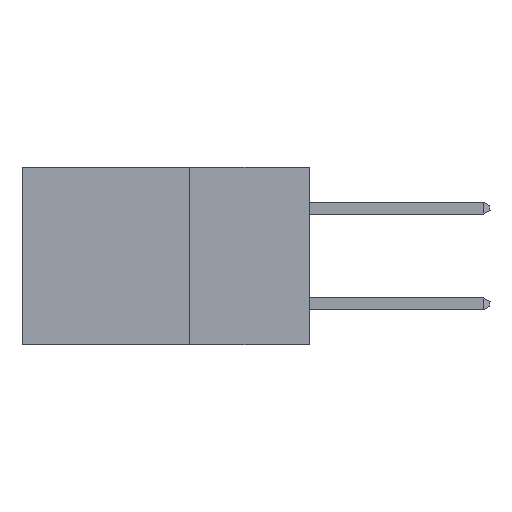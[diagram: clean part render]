
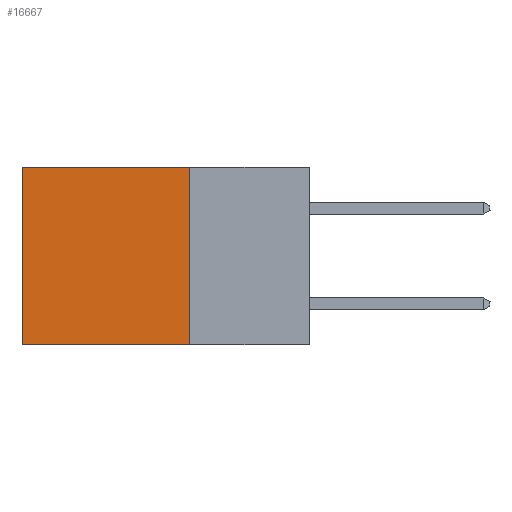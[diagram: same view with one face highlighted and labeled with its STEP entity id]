
A CAD part, left-side view. The second image highlights one B-rep face of the part: STEP entity #16667.
In plain terms, the highlighted planar face has unit normal (-1, 0, 0).
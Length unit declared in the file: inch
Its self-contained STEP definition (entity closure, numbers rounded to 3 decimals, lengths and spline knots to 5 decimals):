
#1924 = DIRECTION ( 'NONE',  ( 0., 0., -1. ) ) ;
#2074 = CARTESIAN_POINT ( 'NONE',  ( 0.2875, 0.25, 0. ) ) ;
#3397 = VECTOR ( 'NONE', #35316, 39.37008 ) ;
#5446 = EDGE_CURVE ( 'NONE', #33733, #5784, #24903, .T. ) ;
#5784 = VERTEX_POINT ( 'NONE', #41349 ) ;
#9668 = DIRECTION ( 'NONE',  ( 1., 0., 0. ) ) ;
#10175 = VECTOR ( 'NONE', #28553, 39.37008 ) ;
#13163 = VECTOR ( 'NONE', #1924, 39.37008 ) ;
#13695 = DIRECTION ( 'NONE',  ( 0., 0., -1. ) ) ;
#14239 = EDGE_CURVE ( 'NONE', #25589, #33733, #38226, .T. ) ;
#14342 = LINE ( 'NONE', #14588, #3397 ) ;
#14551 = CARTESIAN_POINT ( 'NONE',  ( 0.2875, 0.25, -0.37 ) ) ;
#14588 = CARTESIAN_POINT ( 'NONE',  ( 0.2875, 0.25, 0. ) ) ;
#16606 = VERTEX_POINT ( 'NONE', #36648 ) ;
#16667 = ADVANCED_FACE ( 'NONE', ( #27964 ), #26876, .F. ) ;
#24903 = LINE ( 'NONE', #14551, #10175 ) ;
#25589 = VERTEX_POINT ( 'NONE', #40187 ) ;
#26452 = ORIENTED_EDGE ( 'NONE', *, *, #14239, .F. ) ;
#26467 = VECTOR ( 'NONE', #13695, 39.37008 ) ;
#26876 = PLANE ( 'NONE',  #30425 ) ;
#27958 = CARTESIAN_POINT ( 'NONE',  ( 0.2875, 0.25, -0.37 ) ) ;
#27964 = FACE_OUTER_BOUND ( 'NONE', #43372, .T. ) ;
#28553 = DIRECTION ( 'NONE',  ( 0., 1., 0. ) ) ;
#30425 = AXIS2_PLACEMENT_3D ( 'NONE', #44602, #9668, #34052 ) ;
#31067 = ORIENTED_EDGE ( 'NONE', *, *, #34671, .T. ) ;
#33733 = VERTEX_POINT ( 'NONE', #27958 ) ;
#34052 = DIRECTION ( 'NONE',  ( 0., 0., -1. ) ) ;
#34671 = EDGE_CURVE ( 'NONE', #25589, #16606, #14342, .T. ) ;
#35316 = DIRECTION ( 'NONE',  ( 0., 1., 0. ) ) ;
#35597 = EDGE_CURVE ( 'NONE', #16606, #5784, #35739, .T. ) ;
#35739 = LINE ( 'NONE', #45122, #26467 ) ;
#36648 = CARTESIAN_POINT ( 'NONE',  ( 0.2875, 0.6, 0. ) ) ;
#37086 = ORIENTED_EDGE ( 'NONE', *, *, #35597, .T. ) ;
#38226 = LINE ( 'NONE', #2074, #13163 ) ;
#39007 = ORIENTED_EDGE ( 'NONE', *, *, #5446, .F. ) ;
#40187 = CARTESIAN_POINT ( 'NONE',  ( 0.2875, 0.25, 0. ) ) ;
#41349 = CARTESIAN_POINT ( 'NONE',  ( 0.2875, 0.6, -0.37 ) ) ;
#43372 = EDGE_LOOP ( 'NONE', ( #37086, #39007, #26452, #31067 ) ) ;
#44602 = CARTESIAN_POINT ( 'NONE',  ( 0.2875, 0.25, 0. ) ) ;
#45122 = CARTESIAN_POINT ( 'NONE',  ( 0.2875, 0.6, 0. ) ) ;
